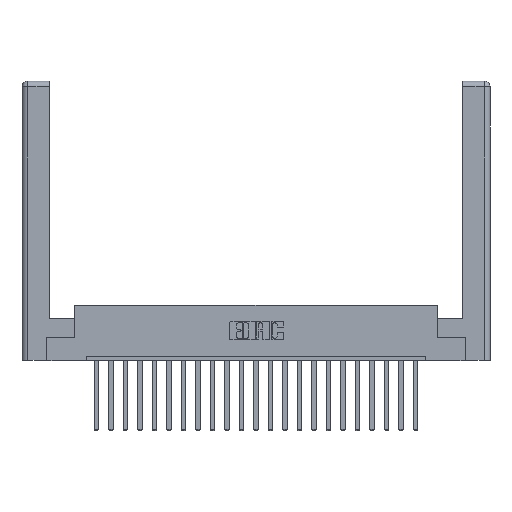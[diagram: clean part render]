
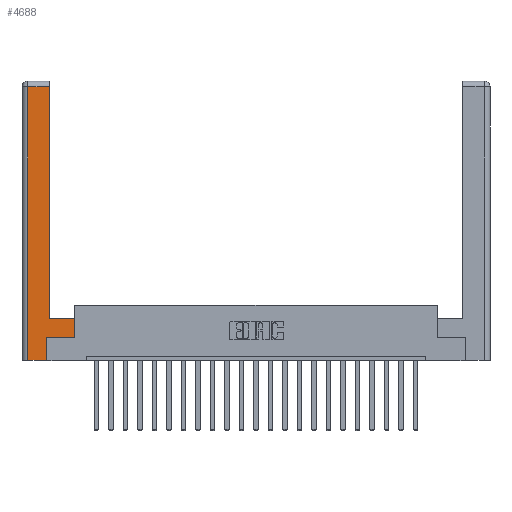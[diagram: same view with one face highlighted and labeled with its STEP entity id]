
A CAD part, top view. The second image highlights one B-rep face of the part: STEP entity #4688.
In plain terms, the highlighted planar face has unit normal (0, 0, 1).
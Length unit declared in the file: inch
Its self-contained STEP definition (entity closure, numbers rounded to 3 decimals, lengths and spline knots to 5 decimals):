
#197 = CARTESIAN_POINT ( 'NONE',  ( 0.295, 3., 0. ) ) ;
#625 = DIRECTION ( 'NONE',  ( 0., 1., 0. ) ) ;
#1038 = LINE ( 'NONE', #1156, #1295 ) ;
#1156 = CARTESIAN_POINT ( 'NONE',  ( 0.265, 0.245, 0. ) ) ;
#1293 = AXIS2_PLACEMENT_3D ( 'NONE', #13716, #15264, #20399 ) ;
#1295 = VECTOR ( 'NONE', #14878, 39.37008 ) ;
#1448 = EDGE_CURVE ( 'NONE', #12725, #20619, #5418, .T. ) ;
#2202 = CARTESIAN_POINT ( 'NONE',  ( 0.565, 0.45, 0. ) ) ;
#2320 = VERTEX_POINT ( 'NONE', #19011 ) ;
#2627 = ORIENTED_EDGE ( 'NONE', *, *, #21708, .T. ) ;
#2695 = CARTESIAN_POINT ( 'NONE',  ( 0.0615, 2.94, 0. ) ) ;
#2700 = EDGE_CURVE ( 'NONE', #15916, #2320, #16491, .T. ) ;
#2715 = DIRECTION ( 'NONE',  ( 0., -1., 0. ) ) ;
#3033 = VECTOR ( 'NONE', #16256, 39.37008 ) ;
#3581 = ORIENTED_EDGE ( 'NONE', *, *, #5820, .T. ) ;
#4436 = ORIENTED_EDGE ( 'NONE', *, *, #2700, .T. ) ;
#4688 = ADVANCED_FACE ( 'NONE', ( #21127 ), #20332, .F. ) ;
#4942 = EDGE_LOOP ( 'NONE', ( #9180, #11752, #2627, #15732, #21443, #4436, #3581, #19107 ) ) ;
#5137 = LINE ( 'NONE', #2202, #5675 ) ;
#5204 = EDGE_CURVE ( 'NONE', #11460, #19774, #10191, .T. ) ;
#5418 = LINE ( 'NONE', #19414, #21619 ) ;
#5675 = VECTOR ( 'NONE', #625, 39.37008 ) ;
#5820 = EDGE_CURVE ( 'NONE', #2320, #12681, #5137, .T. ) ;
#6206 = CARTESIAN_POINT ( 'NONE',  ( 0.265, 0., 0. ) ) ;
#6780 = LINE ( 'NONE', #21275, #10764 ) ;
#7930 = DIRECTION ( 'NONE',  ( 1., 0., 0. ) ) ;
#8669 = VERTEX_POINT ( 'NONE', #13878 ) ;
#9180 = ORIENTED_EDGE ( 'NONE', *, *, #17645, .T. ) ;
#9341 = VECTOR ( 'NONE', #18841, 39.37008 ) ;
#10109 = CARTESIAN_POINT ( 'NONE',  ( 0.565, 0.45, 0. ) ) ;
#10191 = LINE ( 'NONE', #2695, #3033 ) ;
#10764 = VECTOR ( 'NONE', #2715, 39.37008 ) ;
#10771 = VECTOR ( 'NONE', #13239, 39.37008 ) ;
#11460 = VERTEX_POINT ( 'NONE', #20050 ) ;
#11752 = ORIENTED_EDGE ( 'NONE', *, *, #5204, .T. ) ;
#11761 = CARTESIAN_POINT ( 'NONE',  ( 0.265, 0.245, 0. ) ) ;
#12681 = VERTEX_POINT ( 'NONE', #10109 ) ;
#12725 = VERTEX_POINT ( 'NONE', #13578 ) ;
#13239 = DIRECTION ( 'NONE',  ( -1., 0., 0. ) ) ;
#13578 = CARTESIAN_POINT ( 'NONE',  ( 0.0615, 0., 0. ) ) ;
#13716 = CARTESIAN_POINT ( 'NONE',  ( 0., 0., 0. ) ) ;
#13878 = CARTESIAN_POINT ( 'NONE',  ( 0.295, 0.45, 0. ) ) ;
#14498 = EDGE_CURVE ( 'NONE', #20619, #15916, #1038, .T. ) ;
#14878 = DIRECTION ( 'NONE',  ( 0., 1., 0. ) ) ;
#15263 = LINE ( 'NONE', #18600, #10771 ) ;
#15264 = DIRECTION ( 'NONE',  ( 0., 0., -1. ) ) ;
#15732 = ORIENTED_EDGE ( 'NONE', *, *, #1448, .T. ) ;
#15916 = VERTEX_POINT ( 'NONE', #11761 ) ;
#16237 = EDGE_CURVE ( 'NONE', #12681, #8669, #15263, .T. ) ;
#16256 = DIRECTION ( 'NONE',  ( -1., 0., 0. ) ) ;
#16491 = LINE ( 'NONE', #17600, #21018 ) ;
#17525 = DIRECTION ( 'NONE',  ( 1., 0., 0. ) ) ;
#17600 = CARTESIAN_POINT ( 'NONE',  ( 0.565, 0.245, 0. ) ) ;
#17645 = EDGE_CURVE ( 'NONE', #8669, #11460, #20488, .T. ) ;
#18600 = CARTESIAN_POINT ( 'NONE',  ( 0.295, 0.45, 0. ) ) ;
#18841 = DIRECTION ( 'NONE',  ( 0., 1., 0. ) ) ;
#19011 = CARTESIAN_POINT ( 'NONE',  ( 0.565, 0.245, 0. ) ) ;
#19107 = ORIENTED_EDGE ( 'NONE', *, *, #16237, .T. ) ;
#19414 = CARTESIAN_POINT ( 'NONE',  ( 0.265, 0., 0. ) ) ;
#19774 = VERTEX_POINT ( 'NONE', #22011 ) ;
#20050 = CARTESIAN_POINT ( 'NONE',  ( 0.295, 2.94, 0. ) ) ;
#20332 = PLANE ( 'NONE',  #1293 ) ;
#20399 = DIRECTION ( 'NONE',  ( -1., 0., 0. ) ) ;
#20488 = LINE ( 'NONE', #197, #9341 ) ;
#20619 = VERTEX_POINT ( 'NONE', #6206 ) ;
#21018 = VECTOR ( 'NONE', #7930, 39.37008 ) ;
#21127 = FACE_OUTER_BOUND ( 'NONE', #4942, .T. ) ;
#21275 = CARTESIAN_POINT ( 'NONE',  ( 0.0615, 0., 0. ) ) ;
#21443 = ORIENTED_EDGE ( 'NONE', *, *, #14498, .T. ) ;
#21619 = VECTOR ( 'NONE', #17525, 39.37008 ) ;
#21708 = EDGE_CURVE ( 'NONE', #19774, #12725, #6780, .T. ) ;
#22011 = CARTESIAN_POINT ( 'NONE',  ( 0.0615, 2.94, 0. ) ) ;
